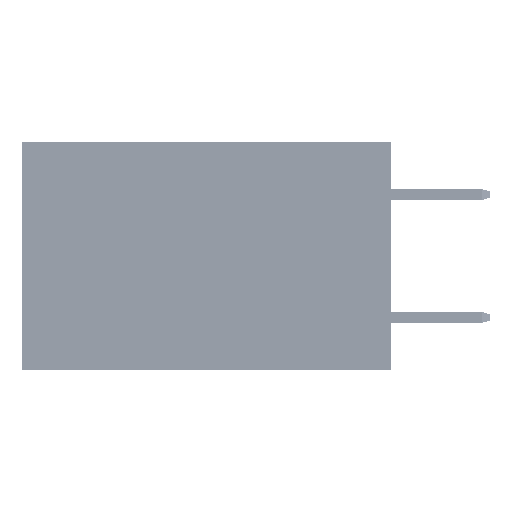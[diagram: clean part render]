
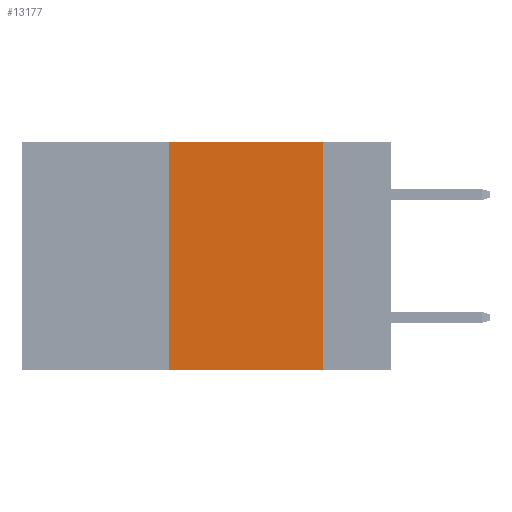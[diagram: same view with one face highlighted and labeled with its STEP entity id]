
A CAD part, left-side view. The second image highlights one B-rep face of the part: STEP entity #13177.
In plain terms, the highlighted planar face has unit normal (-1, 0, 0).
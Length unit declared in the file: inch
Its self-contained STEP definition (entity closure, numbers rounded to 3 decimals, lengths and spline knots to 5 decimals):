
#1471 = FACE_OUTER_BOUND ( 'NONE', #28368, .T. ) ;
#1481 = VERTEX_POINT ( 'NONE', #38612 ) ;
#1727 = PLANE ( 'NONE',  #9717 ) ;
#2193 = LINE ( 'NONE', #33121, #25298 ) ;
#2583 = VERTEX_POINT ( 'NONE', #16688 ) ;
#2738 = ORIENTED_EDGE ( 'NONE', *, *, #46884, .F. ) ;
#4612 = EDGE_CURVE ( 'NONE', #1481, #14241, #44473, .T. ) ;
#5029 = EDGE_CURVE ( 'NONE', #2583, #1481, #9096, .T. ) ;
#8662 = CARTESIAN_POINT ( 'NONE',  ( 0., 0.36, -0.37 ) ) ;
#9096 = LINE ( 'NONE', #48753, #43905 ) ;
#9661 = DIRECTION ( 'NONE',  ( 0., 0., -1. ) ) ;
#9717 = AXIS2_PLACEMENT_3D ( 'NONE', #41103, #36237, #43925 ) ;
#12422 = ORIENTED_EDGE ( 'NONE', *, *, #5029, .F. ) ;
#13177 = ADVANCED_FACE ( 'NONE', ( #1471 ), #1727, .F. ) ;
#14241 = VERTEX_POINT ( 'NONE', #32991 ) ;
#15918 = VERTEX_POINT ( 'NONE', #8662 ) ;
#16688 = CARTESIAN_POINT ( 'NONE',  ( 0., 0.36, 0. ) ) ;
#18074 = VECTOR ( 'NONE', #9661, 39.37008 ) ;
#20779 = VECTOR ( 'NONE', #26954, 39.37008 ) ;
#24664 = DIRECTION ( 'NONE',  ( 0., -1., 0. ) ) ;
#25149 = DIRECTION ( 'NONE',  ( 0., -1., 0. ) ) ;
#25298 = VECTOR ( 'NONE', #25149, 39.37008 ) ;
#26465 = CARTESIAN_POINT ( 'NONE',  ( 0., 0.36, 0. ) ) ;
#26954 = DIRECTION ( 'NONE',  ( 0., 0., 1. ) ) ;
#27784 = EDGE_CURVE ( 'NONE', #15918, #14241, #2193, .T. ) ;
#28368 = EDGE_LOOP ( 'NONE', ( #50297, #12422, #2738, #35926 ) ) ;
#28563 = CARTESIAN_POINT ( 'NONE',  ( 0., 0.11, 0. ) ) ;
#32991 = CARTESIAN_POINT ( 'NONE',  ( 0., 0.11, -0.37 ) ) ;
#33121 = CARTESIAN_POINT ( 'NONE',  ( 0., 0.6, -0.37 ) ) ;
#35926 = ORIENTED_EDGE ( 'NONE', *, *, #27784, .T. ) ;
#36237 = DIRECTION ( 'NONE',  ( 1., 0., 0. ) ) ;
#38612 = CARTESIAN_POINT ( 'NONE',  ( 0., 0.11, 0. ) ) ;
#41103 = CARTESIAN_POINT ( 'NONE',  ( 0., 0.6, 0. ) ) ;
#42856 = LINE ( 'NONE', #26465, #20779 ) ;
#43905 = VECTOR ( 'NONE', #24664, 39.37008 ) ;
#43925 = DIRECTION ( 'NONE',  ( 0., 0., -1. ) ) ;
#44473 = LINE ( 'NONE', #28563, #18074 ) ;
#46884 = EDGE_CURVE ( 'NONE', #15918, #2583, #42856, .T. ) ;
#48753 = CARTESIAN_POINT ( 'NONE',  ( 0., 0.6, 0. ) ) ;
#50297 = ORIENTED_EDGE ( 'NONE', *, *, #4612, .F. ) ;
